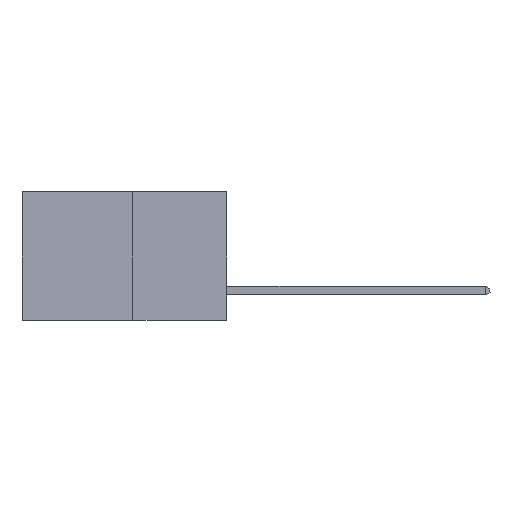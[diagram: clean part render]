
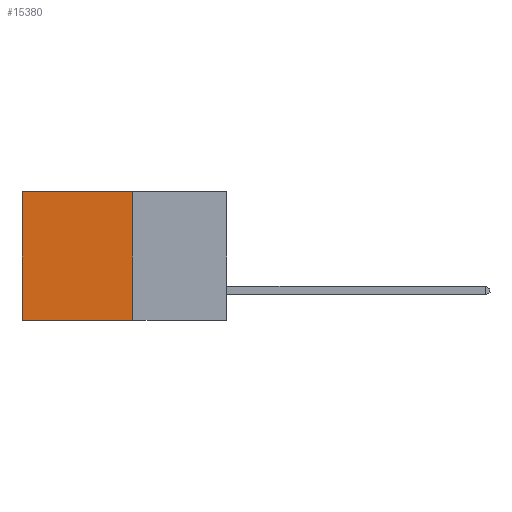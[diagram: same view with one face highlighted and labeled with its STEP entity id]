
A CAD part, left-side view. The second image highlights one B-rep face of the part: STEP entity #15380.
In plain terms, the highlighted planar face has unit normal (-1, 0, 0).
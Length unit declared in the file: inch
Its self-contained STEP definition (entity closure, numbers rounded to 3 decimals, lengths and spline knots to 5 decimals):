
#800 = VECTOR ( 'NONE', #13894, 39.37008 ) ;
#1565 = LINE ( 'NONE', #5494, #7571 ) ;
#1771 = DIRECTION ( 'NONE',  ( 0., 0., -1. ) ) ;
#1840 = AXIS2_PLACEMENT_3D ( 'NONE', #11906, #9414, #1771 ) ;
#2282 = CARTESIAN_POINT ( 'NONE',  ( 0.277, 0.27, -0.37 ) ) ;
#3356 = ORIENTED_EDGE ( 'NONE', *, *, #16083, .T. ) ;
#3818 = CARTESIAN_POINT ( 'NONE',  ( 0.277, 0.59, -0.37 ) ) ;
#4580 = ORIENTED_EDGE ( 'NONE', *, *, #11051, .F. ) ;
#4893 = DIRECTION ( 'NONE',  ( 0., 0., -1. ) ) ;
#4983 = CARTESIAN_POINT ( 'NONE',  ( 0.277, 0.27, 0. ) ) ;
#5494 = CARTESIAN_POINT ( 'NONE',  ( 0.277, 0.59, -0.37 ) ) ;
#6483 = DIRECTION ( 'NONE',  ( 0., 1., 0. ) ) ;
#6540 = CARTESIAN_POINT ( 'NONE',  ( 0.277, 0.27, 0. ) ) ;
#7158 = ORIENTED_EDGE ( 'NONE', *, *, #14478, .F. ) ;
#7350 = VERTEX_POINT ( 'NONE', #3818 ) ;
#7458 = VERTEX_POINT ( 'NONE', #14084 ) ;
#7571 = VECTOR ( 'NONE', #15479, 39.37008 ) ;
#7633 = LINE ( 'NONE', #15094, #800 ) ;
#7920 = VECTOR ( 'NONE', #4893, 39.37008 ) ;
#9414 = DIRECTION ( 'NONE',  ( 1., 0., 0. ) ) ;
#9551 = LINE ( 'NONE', #6540, #12877 ) ;
#10824 = VERTEX_POINT ( 'NONE', #13244 ) ;
#11051 = EDGE_CURVE ( 'NONE', #11772, #10824, #14566, .T. ) ;
#11298 = ORIENTED_EDGE ( 'NONE', *, *, #15992, .T. ) ;
#11772 = VERTEX_POINT ( 'NONE', #4983 ) ;
#11906 = CARTESIAN_POINT ( 'NONE',  ( 0.277, 0.27, -0.37 ) ) ;
#12711 = FACE_OUTER_BOUND ( 'NONE', #14848, .T. ) ;
#12877 = VECTOR ( 'NONE', #6483, 39.37008 ) ;
#13128 = PLANE ( 'NONE',  #1840 ) ;
#13244 = CARTESIAN_POINT ( 'NONE',  ( 0.277, 0.27, -0.37 ) ) ;
#13894 = DIRECTION ( 'NONE',  ( 0., 1., 0. ) ) ;
#14084 = CARTESIAN_POINT ( 'NONE',  ( 0.277, 0.59, 0. ) ) ;
#14478 = EDGE_CURVE ( 'NONE', #10824, #7350, #7633, .T. ) ;
#14566 = LINE ( 'NONE', #2282, #7920 ) ;
#14848 = EDGE_LOOP ( 'NONE', ( #3356, #7158, #4580, #11298 ) ) ;
#15094 = CARTESIAN_POINT ( 'NONE',  ( 0.277, 0.27, -0.37 ) ) ;
#15380 = ADVANCED_FACE ( 'NONE', ( #12711 ), #13128, .F. ) ;
#15479 = DIRECTION ( 'NONE',  ( 0., 0., -1. ) ) ;
#15992 = EDGE_CURVE ( 'NONE', #11772, #7458, #9551, .T. ) ;
#16083 = EDGE_CURVE ( 'NONE', #7458, #7350, #1565, .T. ) ;
